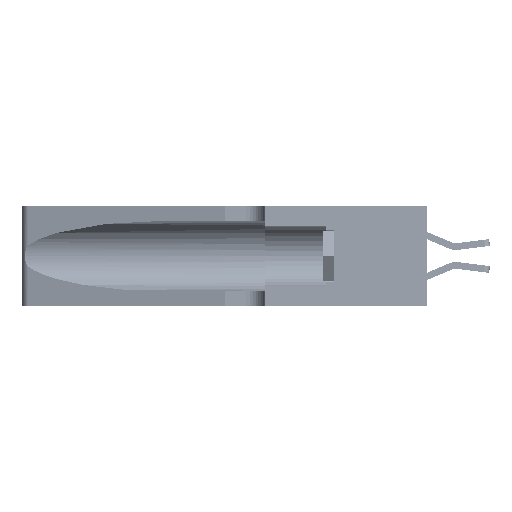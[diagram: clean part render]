
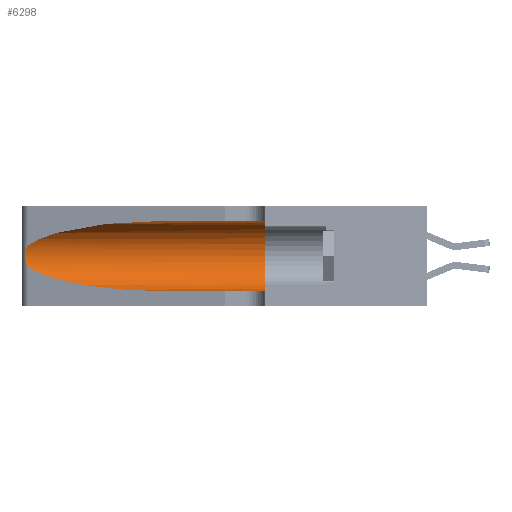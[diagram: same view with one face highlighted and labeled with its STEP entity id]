
A CAD part, left-side view. The second image highlights one B-rep face of the part: STEP entity #6298.
In plain terms, the highlighted cylindrical face has radius 3.308 mm (diameter 6.617 mm), a partial arc.
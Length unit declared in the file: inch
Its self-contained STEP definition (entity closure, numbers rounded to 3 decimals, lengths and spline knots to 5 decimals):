
#1345 = ORIENTED_EDGE ( 'NONE', *, *, #50082, .T. ) ;
#1658 = LINE ( 'NONE', #39297, #32467 ) ;
#2585 = CARTESIAN_POINT ( 'NONE',  ( 0.1305, 0.72297, 0.31525 ) ) ;
#3467 = AXIS2_PLACEMENT_3D ( 'NONE', #50809, #21588, #5878 ) ;
#3677 = EDGE_CURVE ( 'NONE', #39200, #43557, #9662, .T. ) ;
#4629 = B_SPLINE_CURVE_WITH_KNOTS ( 'NONE', 3,
 ( #29086, #41789, #21336, #45564, #25464, #9242, #37858, #9588, #38378, #38554, #50370, #14016, #9412, #34621 ),
 .UNSPECIFIED., .F., .F.,
 ( 4, 2, 2, 2, 2, 2, 4 ),
 ( 0., 0.00027, 0.00053, 0.00107, 0.0016, 0.00187, 0.00214 ),
 .UNSPECIFIED. ) ;
#4960 = CARTESIAN_POINT ( 'NONE',  ( 0.1305, 0.72297, 0.05475 ) ) ;
#5411 = VERTEX_POINT ( 'NONE', #47196 ) ;
#5878 = DIRECTION ( 'NONE',  ( 0., 0., 1. ) ) ;
#6298 = ADVANCED_FACE ( 'NONE', ( #17643 ), #49044, .F. ) ;
#7398 = DIRECTION ( 'NONE',  ( 0., -1., 0. ) ) ;
#8841 = ORIENTED_EDGE ( 'NONE', *, *, #11230, .T. ) ;
#8927 = CARTESIAN_POINT ( 'NONE',  ( 0.2373, 1.15595, 0.08982 ) ) ;
#9242 = CARTESIAN_POINT ( 'NONE',  ( 0.26018, 1.23835, 0.19895 ) ) ;
#9412 = CARTESIAN_POINT ( 'NONE',  ( 0.25555, 1.22993, 0.14849 ) ) ;
#9588 = CARTESIAN_POINT ( 'NONE',  ( 0.26075, 1.23896, 0.178 ) ) ;
#9662 = LINE ( 'NONE', #37227, #16070 ) ;
#11230 = EDGE_CURVE ( 'NONE', #49634, #47766, #1658, .T. ) ;
#12864 = EDGE_CURVE ( 'NONE', #5411, #49634, #50573, .T. ) ;
#14016 = CARTESIAN_POINT ( 'NONE',  ( 0.25639, 1.23186, 0.15144 ) ) ;
#14683 = CARTESIAN_POINT ( 'NONE',  ( 0.25487, 1.22718, 0.22369 ) ) ;
#16070 = VECTOR ( 'NONE', #41315, 39.37008 ) ;
#16745 = CARTESIAN_POINT ( 'NONE',  ( 0.1305, 0.72297, 0.31525 ) ) ;
#17643 = FACE_OUTER_BOUND ( 'NONE', #39144, .T. ) ;
#18982 = DIRECTION ( 'NONE',  ( 0., 0., -1. ) ) ;
#21336 = CARTESIAN_POINT ( 'NONE',  ( 0.25639, 1.23184, 0.21858 ) ) ;
#21588 = DIRECTION ( 'NONE',  ( 0., 1., 0. ) ) ;
#22929 = ORIENTED_EDGE ( 'NONE', *, *, #12864, .T. ) ;
#24642 = CARTESIAN_POINT ( 'NONE',  ( 0.1305, 0.35, 0.31525 ) ) ;
#25136 = VERTEX_POINT ( 'NONE', #14683 ) ;
#25464 = CARTESIAN_POINT ( 'NONE',  ( 0.25854, 1.2359, 0.20912 ) ) ;
#26677 = ORIENTED_EDGE ( 'NONE', *, *, #32856, .F. ) ;
#29086 = CARTESIAN_POINT ( 'NONE',  ( 0.25487, 1.22718, 0.22369 ) ) ;
#29307 = EDGE_CURVE ( 'NONE', #39200, #25136, #44341, .T. ) ;
#29480 = CARTESIAN_POINT ( 'NONE',  ( 0.18966, 0.96281, 0.05475 ) ) ;
#31739 = CARTESIAN_POINT ( 'NONE',  ( 0.1305, 1.61858, 0.185 ) ) ;
#32467 = VECTOR ( 'NONE', #39469, 39.37008 ) ;
#32856 = EDGE_CURVE ( 'NONE', #43557, #47766, #38780, .T. ) ;
#33943 = CARTESIAN_POINT ( 'NONE',  ( 0.25487, 1.22718, 0.14631 ) ) ;
#34621 = CARTESIAN_POINT ( 'NONE',  ( 0.25487, 1.22718, 0.14631 ) ) ;
#34833 = CARTESIAN_POINT ( 'NONE',  ( 0.2373, 1.15595, 0.28018 ) ) ;
#37227 = CARTESIAN_POINT ( 'NONE',  ( 0.1305, 1.61858, 0.31525 ) ) ;
#37858 = CARTESIAN_POINT ( 'NONE',  ( 0.26075, 1.23896, 0.19203 ) ) ;
#38378 = CARTESIAN_POINT ( 'NONE',  ( 0.26017, 1.23833, 0.17102 ) ) ;
#38554 = CARTESIAN_POINT ( 'NONE',  ( 0.25856, 1.23593, 0.16098 ) ) ;
#38780 = CIRCLE ( 'NONE', #3467, 0.13025 ) ;
#38958 = ORIENTED_EDGE ( 'NONE', *, *, #3677, .F. ) ;
#39144 = EDGE_LOOP ( 'NONE', ( #39570, #1345, #22929, #8841, #26677, #38958 ) ) ;
#39200 = VERTEX_POINT ( 'NONE', #16745 ) ;
#39297 = CARTESIAN_POINT ( 'NONE',  ( 0.1305, 1.61858, 0.05475 ) ) ;
#39469 = DIRECTION ( 'NONE',  ( 0., -1., 0. ) ) ;
#39570 = ORIENTED_EDGE ( 'NONE', *, *, #29307, .T. ) ;
#41315 = DIRECTION ( 'NONE',  ( 0., -1., 0. ) ) ;
#41789 = CARTESIAN_POINT ( 'NONE',  ( 0.25555, 1.22994, 0.2215 ) ) ;
#42691 = CARTESIAN_POINT ( 'NONE',  ( 0.18966, 0.96281, 0.31525 ) ) ;
#43557 = VERTEX_POINT ( 'NONE', #24642 ) ;
#43572 = CARTESIAN_POINT ( 'NONE',  ( 0.1305, 0.35, 0.05475 ) ) ;
#44341 =( BOUNDED_CURVE ( )  B_SPLINE_CURVE ( 3, ( #2585, #42691, #34833, #51456 ),
 .UNSPECIFIED., .F., .T. ) 
 B_SPLINE_CURVE_WITH_KNOTS ( ( 4, 4 ),
 ( 1.5708, 2.84003 ),
 .UNSPECIFIED. ) 
 CURVE ( )  GEOMETRIC_REPRESENTATION_ITEM ( )  RATIONAL_B_SPLINE_CURVE ( ( 1., 0.87, 0.87, 1. ) ) 
 REPRESENTATION_ITEM ( '' )  );
#45564 = CARTESIAN_POINT ( 'NONE',  ( 0.25787, 1.23484, 0.2124 ) ) ;
#47196 = CARTESIAN_POINT ( 'NONE',  ( 0.25487, 1.22718, 0.14631 ) ) ;
#47766 = VERTEX_POINT ( 'NONE', #43572 ) ;
#48270 = CARTESIAN_POINT ( 'NONE',  ( 0.1305, 0.72297, 0.05475 ) ) ;
#49044 = CYLINDRICAL_SURFACE ( 'NONE', #51095, 0.13025 ) ;
#49634 = VERTEX_POINT ( 'NONE', #48270 ) ;
#50082 = EDGE_CURVE ( 'NONE', #25136, #5411, #4629, .T. ) ;
#50370 = CARTESIAN_POINT ( 'NONE',  ( 0.25789, 1.23486, 0.15765 ) ) ;
#50573 =( BOUNDED_CURVE ( )  B_SPLINE_CURVE ( 3, ( #33943, #8927, #29480, #4960 ),
 .UNSPECIFIED., .F., .F. ) 
 B_SPLINE_CURVE_WITH_KNOTS ( ( 4, 4 ),
 ( 3.44316, 4.71239 ),
 .UNSPECIFIED. ) 
 CURVE ( )  GEOMETRIC_REPRESENTATION_ITEM ( )  RATIONAL_B_SPLINE_CURVE ( ( 1., 0.87, 0.87, 1. ) ) 
 REPRESENTATION_ITEM ( '' )  );
#50809 = CARTESIAN_POINT ( 'NONE',  ( 0.1305, 0.35, 0.185 ) ) ;
#51095 = AXIS2_PLACEMENT_3D ( 'NONE', #31739, #7398, #18982 ) ;
#51456 = CARTESIAN_POINT ( 'NONE',  ( 0.25487, 1.22718, 0.22369 ) ) ;
